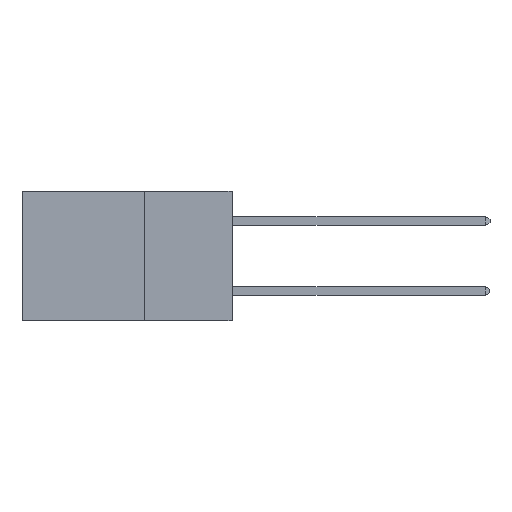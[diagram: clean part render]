
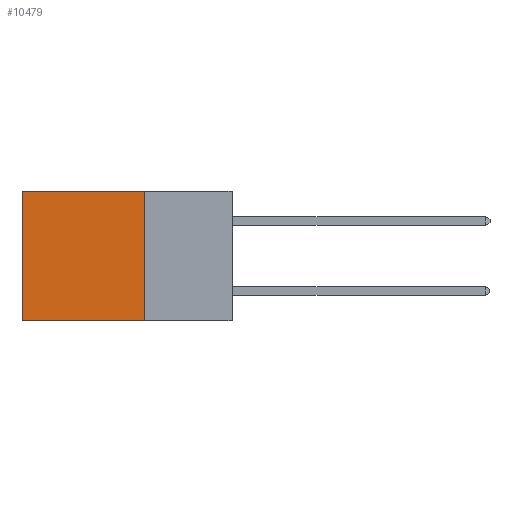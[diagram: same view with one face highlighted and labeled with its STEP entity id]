
A CAD part, left-side view. The second image highlights one B-rep face of the part: STEP entity #10479.
In plain terms, the highlighted planar face has unit normal (-1, 0, 0).
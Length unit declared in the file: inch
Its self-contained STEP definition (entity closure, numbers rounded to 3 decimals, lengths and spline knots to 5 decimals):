
#374 = CARTESIAN_POINT ( 'NONE',  ( 0.2875, 0.6, 0. ) ) ;
#1129 = LINE ( 'NONE', #8228, #10120 ) ;
#1900 = VECTOR ( 'NONE', #5854, 39.37008 ) ;
#2177 = ORIENTED_EDGE ( 'NONE', *, *, #17916, .T. ) ;
#4173 = EDGE_CURVE ( 'NONE', #14565, #10949, #1129, .T. ) ;
#4704 = CARTESIAN_POINT ( 'NONE',  ( 0.2875, 0.25, 0. ) ) ;
#5221 = CARTESIAN_POINT ( 'NONE',  ( 0.2875, 0.25, 0. ) ) ;
#5854 = DIRECTION ( 'NONE',  ( 0., 0., -1. ) ) ;
#6020 = VECTOR ( 'NONE', #8329, 39.37008 ) ;
#6607 = ORIENTED_EDGE ( 'NONE', *, *, #20905, .T. ) ;
#6968 = EDGE_LOOP ( 'NONE', ( #2177, #21295, #21436, #6607 ) ) ;
#8228 = CARTESIAN_POINT ( 'NONE',  ( 0.2875, 0.25, -0.37 ) ) ;
#8329 = DIRECTION ( 'NONE',  ( 0., 0., -1. ) ) ;
#10120 = VECTOR ( 'NONE', #15059, 39.37008 ) ;
#10305 = DIRECTION ( 'NONE',  ( 1., 0., 0. ) ) ;
#10479 = ADVANCED_FACE ( 'NONE', ( #17450 ), #15362, .F. ) ;
#10850 = LINE ( 'NONE', #374, #1900 ) ;
#10949 = VERTEX_POINT ( 'NONE', #16637 ) ;
#11207 = LINE ( 'NONE', #4704, #6020 ) ;
#12722 = CARTESIAN_POINT ( 'NONE',  ( 0.2875, 0.6, 0. ) ) ;
#13992 = VERTEX_POINT ( 'NONE', #21880 ) ;
#14565 = VERTEX_POINT ( 'NONE', #14850 ) ;
#14850 = CARTESIAN_POINT ( 'NONE',  ( 0.2875, 0.25, -0.37 ) ) ;
#15059 = DIRECTION ( 'NONE',  ( 0., 1., 0. ) ) ;
#15169 = VERTEX_POINT ( 'NONE', #12722 ) ;
#15362 = PLANE ( 'NONE',  #16826 ) ;
#16305 = VECTOR ( 'NONE', #20694, 39.37008 ) ;
#16637 = CARTESIAN_POINT ( 'NONE',  ( 0.2875, 0.6, -0.37 ) ) ;
#16826 = AXIS2_PLACEMENT_3D ( 'NONE', #20441, #10305, #22125 ) ;
#16864 = LINE ( 'NONE', #5221, #16305 ) ;
#17450 = FACE_OUTER_BOUND ( 'NONE', #6968, .T. ) ;
#17916 = EDGE_CURVE ( 'NONE', #15169, #10949, #10850, .T. ) ;
#20441 = CARTESIAN_POINT ( 'NONE',  ( 0.2875, 0.25, 0. ) ) ;
#20694 = DIRECTION ( 'NONE',  ( 0., 1., 0. ) ) ;
#20905 = EDGE_CURVE ( 'NONE', #13992, #15169, #16864, .T. ) ;
#21295 = ORIENTED_EDGE ( 'NONE', *, *, #4173, .F. ) ;
#21353 = EDGE_CURVE ( 'NONE', #13992, #14565, #11207, .T. ) ;
#21436 = ORIENTED_EDGE ( 'NONE', *, *, #21353, .F. ) ;
#21880 = CARTESIAN_POINT ( 'NONE',  ( 0.2875, 0.25, 0. ) ) ;
#22125 = DIRECTION ( 'NONE',  ( 0., 0., -1. ) ) ;
